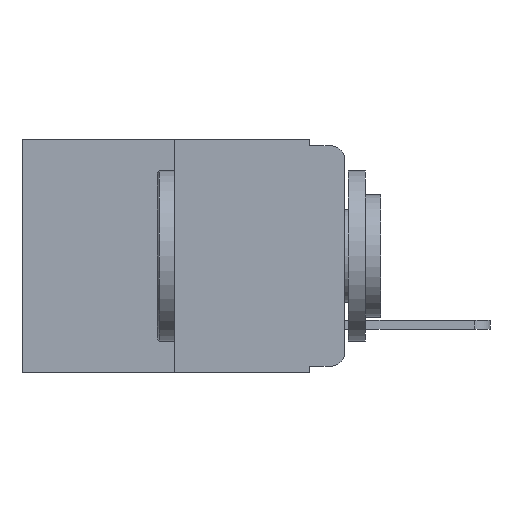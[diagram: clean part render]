
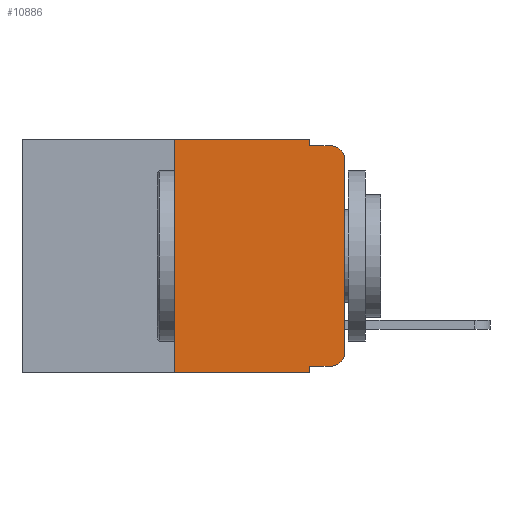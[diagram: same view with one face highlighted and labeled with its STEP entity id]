
A CAD part, left-side view. The second image highlights one B-rep face of the part: STEP entity #10886.
In plain terms, the highlighted planar face has unit normal (-1, 0, 0).
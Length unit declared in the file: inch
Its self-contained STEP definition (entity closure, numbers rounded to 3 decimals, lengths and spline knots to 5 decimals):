
#154 = LINE ( 'NONE', #8524, #11178 ) ;
#461 = VERTEX_POINT ( 'NONE', #12359 ) ;
#616 = EDGE_LOOP ( 'NONE', ( #1111, #1426, #1741, #1314, #9404, #9093, #8785, #7833, #7307, #6082 ) ) ;
#806 = DIRECTION ( 'NONE',  ( 0., 0., 1. ) ) ;
#1111 = ORIENTED_EDGE ( 'NONE', *, *, #3246, .T. ) ;
#1314 = ORIENTED_EDGE ( 'NONE', *, *, #5342, .F. ) ;
#1426 = ORIENTED_EDGE ( 'NONE', *, *, #3849, .T. ) ;
#1441 = CARTESIAN_POINT ( 'NONE',  ( 0., 0.02, -0.313 ) ) ;
#1741 = ORIENTED_EDGE ( 'NONE', *, *, #4920, .F. ) ;
#1858 = VERTEX_POINT ( 'NONE', #4253 ) ;
#2065 = EDGE_CURVE ( 'NONE', #7817, #13142, #12769, .T. ) ;
#2112 = LINE ( 'NONE', #13210, #7274 ) ;
#2438 = LINE ( 'NONE', #4672, #7892 ) ;
#2506 = CARTESIAN_POINT ( 'NONE',  ( 0., 0.051, -0.333 ) ) ;
#2622 = DIRECTION ( 'NONE',  ( 0., 0., -1. ) ) ;
#2773 = CARTESIAN_POINT ( 'NONE',  ( 0., 0., -0.313 ) ) ;
#3246 = EDGE_CURVE ( 'NONE', #6368, #8437, #2112, .T. ) ;
#3453 = AXIS2_PLACEMENT_3D ( 'NONE', #9028, #11860, #6003 ) ;
#3692 = LINE ( 'NONE', #12234, #6591 ) ;
#3790 = PLANE ( 'NONE',  #3453 ) ;
#3849 = EDGE_CURVE ( 'NONE', #8437, #9509, #11926, .T. ) ;
#3853 = CARTESIAN_POINT ( 'NONE',  ( 0., 0., -0.03 ) ) ;
#4248 = LINE ( 'NONE', #11091, #11918 ) ;
#4253 = CARTESIAN_POINT ( 'NONE',  ( 0., 0.02, -0.333 ) ) ;
#4580 = LINE ( 'NONE', #4595, #9722 ) ;
#4595 = CARTESIAN_POINT ( 'NONE',  ( 0., 0.051, -0.333 ) ) ;
#4672 = CARTESIAN_POINT ( 'NONE',  ( 0., 0.473, -0.343 ) ) ;
#4917 = DIRECTION ( 'NONE',  ( -1., 0., 0. ) ) ;
#4918 = VECTOR ( 'NONE', #10143, 39.37008 ) ;
#4920 = EDGE_CURVE ( 'NONE', #12351, #9509, #4248, .T. ) ;
#5286 = LINE ( 'NONE', #13362, #4918 ) ;
#5342 = EDGE_CURVE ( 'NONE', #13142, #12351, #5286, .T. ) ;
#5449 = DIRECTION ( 'NONE',  ( 0., 0., -1. ) ) ;
#5759 = DIRECTION ( 'NONE',  ( 0., -1., 0. ) ) ;
#5763 = CIRCLE ( 'NONE', #7656, 0.02 ) ;
#5847 = EDGE_CURVE ( 'NONE', #461, #7817, #3692, .T. ) ;
#5862 = CARTESIAN_POINT ( 'NONE',  ( 0., 0.051, -0.01 ) ) ;
#5871 = EDGE_CURVE ( 'NONE', #9653, #8018, #154, .T. ) ;
#6003 = DIRECTION ( 'NONE',  ( 0., 0., -1. ) ) ;
#6082 = ORIENTED_EDGE ( 'NONE', *, *, #6285, .T. ) ;
#6116 = EDGE_CURVE ( 'NONE', #9653, #1858, #4580, .T. ) ;
#6285 = EDGE_CURVE ( 'NONE', #1858, #6368, #5763, .T. ) ;
#6330 = DIRECTION ( 'NONE',  ( 0., -1., 0. ) ) ;
#6368 = VERTEX_POINT ( 'NONE', #2773 ) ;
#6591 = VECTOR ( 'NONE', #806, 39.37008 ) ;
#6796 = CARTESIAN_POINT ( 'NONE',  ( 0., 0.473, 0. ) ) ;
#6877 = CARTESIAN_POINT ( 'NONE',  ( 0., 0.02, -0.03 ) ) ;
#7078 = DIRECTION ( 'NONE',  ( 0., 0., 1. ) ) ;
#7274 = VECTOR ( 'NONE', #7078, 39.37008 ) ;
#7307 = ORIENTED_EDGE ( 'NONE', *, *, #6116, .T. ) ;
#7656 = AXIS2_PLACEMENT_3D ( 'NONE', #1441, #9030, #2622 ) ;
#7817 = VERTEX_POINT ( 'NONE', #10436 ) ;
#7833 = ORIENTED_EDGE ( 'NONE', *, *, #5871, .F. ) ;
#7892 = VECTOR ( 'NONE', #5759, 39.37008 ) ;
#8018 = VERTEX_POINT ( 'NONE', #11485 ) ;
#8437 = VERTEX_POINT ( 'NONE', #3853 ) ;
#8524 = CARTESIAN_POINT ( 'NONE',  ( 0., 0.051, 0. ) ) ;
#8779 = DIRECTION ( 'NONE',  ( 0., -1., 0. ) ) ;
#8785 = ORIENTED_EDGE ( 'NONE', *, *, #9563, .T. ) ;
#9028 = CARTESIAN_POINT ( 'NONE',  ( 0., 0.473, 0. ) ) ;
#9030 = DIRECTION ( 'NONE',  ( -1., 0., 0. ) ) ;
#9093 = ORIENTED_EDGE ( 'NONE', *, *, #5847, .F. ) ;
#9404 = ORIENTED_EDGE ( 'NONE', *, *, #2065, .F. ) ;
#9509 = VERTEX_POINT ( 'NONE', #11582 ) ;
#9563 = EDGE_CURVE ( 'NONE', #461, #8018, #2438, .T. ) ;
#9653 = VERTEX_POINT ( 'NONE', #2506 ) ;
#9722 = VECTOR ( 'NONE', #8779, 39.37008 ) ;
#9818 = CARTESIAN_POINT ( 'NONE',  ( 0., 0.051, 0. ) ) ;
#10143 = DIRECTION ( 'NONE',  ( 0., 0., -1. ) ) ;
#10406 = VECTOR ( 'NONE', #6330, 39.37008 ) ;
#10423 = AXIS2_PLACEMENT_3D ( 'NONE', #6877, #4917, #13177 ) ;
#10436 = CARTESIAN_POINT ( 'NONE',  ( 0., 0.25, 0. ) ) ;
#10860 = DIRECTION ( 'NONE',  ( 0., -1., 0. ) ) ;
#10886 = ADVANCED_FACE ( 'NONE', ( #13055 ), #3790, .F. ) ;
#11091 = CARTESIAN_POINT ( 'NONE',  ( 0., 0.051, -0.01 ) ) ;
#11178 = VECTOR ( 'NONE', #5449, 39.37008 ) ;
#11485 = CARTESIAN_POINT ( 'NONE',  ( 0., 0.051, -0.343 ) ) ;
#11582 = CARTESIAN_POINT ( 'NONE',  ( 0., 0.02, -0.01 ) ) ;
#11860 = DIRECTION ( 'NONE',  ( 1., 0., 0. ) ) ;
#11918 = VECTOR ( 'NONE', #10860, 39.37008 ) ;
#11926 = CIRCLE ( 'NONE', #10423, 0.02 ) ;
#12234 = CARTESIAN_POINT ( 'NONE',  ( 0., 0.25, 0. ) ) ;
#12351 = VERTEX_POINT ( 'NONE', #5862 ) ;
#12359 = CARTESIAN_POINT ( 'NONE',  ( 0., 0.25, -0.343 ) ) ;
#12769 = LINE ( 'NONE', #6796, #10406 ) ;
#13055 = FACE_OUTER_BOUND ( 'NONE', #616, .T. ) ;
#13142 = VERTEX_POINT ( 'NONE', #9818 ) ;
#13177 = DIRECTION ( 'NONE',  ( 0., 0., -1. ) ) ;
#13210 = CARTESIAN_POINT ( 'NONE',  ( 0., 0., 0. ) ) ;
#13362 = CARTESIAN_POINT ( 'NONE',  ( 0., 0.051, 0. ) ) ;
